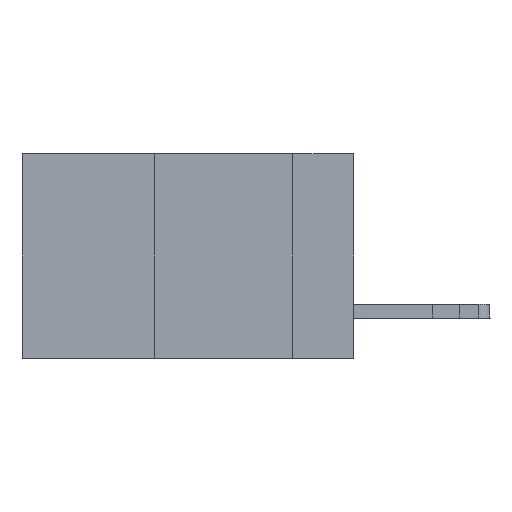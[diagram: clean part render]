
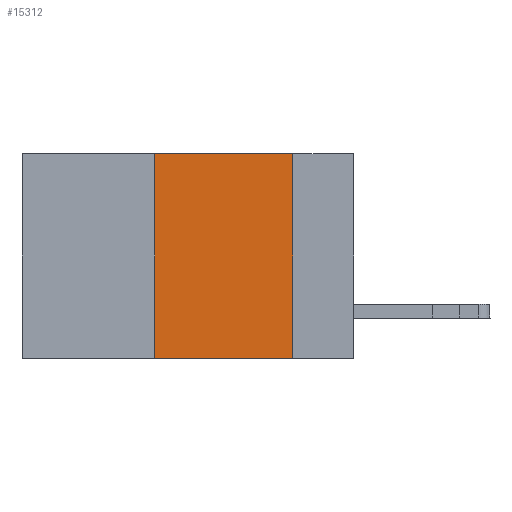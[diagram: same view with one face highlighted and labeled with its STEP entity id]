
A CAD part, left-side view. The second image highlights one B-rep face of the part: STEP entity #15312.
In plain terms, the highlighted planar face has unit normal (-1, 0, 0).
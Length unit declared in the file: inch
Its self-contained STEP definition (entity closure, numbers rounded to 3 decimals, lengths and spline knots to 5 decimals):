
#2094 = DIRECTION ( 'NONE',  ( 1., 0., 0. ) ) ;
#3009 = CARTESIAN_POINT ( 'NONE',  ( 0., 0.11, 0. ) ) ;
#3119 = VECTOR ( 'NONE', #15580, 39.37008 ) ;
#3267 = LINE ( 'NONE', #10671, #11574 ) ;
#3893 = ORIENTED_EDGE ( 'NONE', *, *, #8910, .F. ) ;
#4150 = CARTESIAN_POINT ( 'NONE',  ( 0., 0.6, -0.37 ) ) ;
#4875 = VECTOR ( 'NONE', #9356, 39.37008 ) ;
#5957 = VERTEX_POINT ( 'NONE', #6517 ) ;
#6417 = EDGE_CURVE ( 'NONE', #9310, #8151, #13589, .T. ) ;
#6464 = CARTESIAN_POINT ( 'NONE',  ( 0., 0.36, -0.37 ) ) ;
#6517 = CARTESIAN_POINT ( 'NONE',  ( 0., 0.36, 0. ) ) ;
#7467 = CARTESIAN_POINT ( 'NONE',  ( 0., 0.11, 0. ) ) ;
#8151 = VERTEX_POINT ( 'NONE', #9214 ) ;
#8866 = ORIENTED_EDGE ( 'NONE', *, *, #16537, .F. ) ;
#8910 = EDGE_CURVE ( 'NONE', #5957, #9310, #12838, .T. ) ;
#9214 = CARTESIAN_POINT ( 'NONE',  ( 0., 0.11, -0.37 ) ) ;
#9310 = VERTEX_POINT ( 'NONE', #7467 ) ;
#9356 = DIRECTION ( 'NONE',  ( 0., 0., -1. ) ) ;
#9537 = CARTESIAN_POINT ( 'NONE',  ( 0., 0.6, 0. ) ) ;
#9902 = ORIENTED_EDGE ( 'NONE', *, *, #14294, .T. ) ;
#10671 = CARTESIAN_POINT ( 'NONE',  ( 0., 0.36, 0. ) ) ;
#11574 = VECTOR ( 'NONE', #12287, 39.37008 ) ;
#12052 = CARTESIAN_POINT ( 'NONE',  ( 0., 0.6, 0. ) ) ;
#12287 = DIRECTION ( 'NONE',  ( 0., 0., 1. ) ) ;
#12838 = LINE ( 'NONE', #9537, #16549 ) ;
#13589 = LINE ( 'NONE', #3009, #4875 ) ;
#13662 = DIRECTION ( 'NONE',  ( 0., 0., -1. ) ) ;
#14294 = EDGE_CURVE ( 'NONE', #14515, #8151, #15181, .T. ) ;
#14385 = DIRECTION ( 'NONE',  ( 0., -1., 0. ) ) ;
#14515 = VERTEX_POINT ( 'NONE', #6464 ) ;
#15181 = LINE ( 'NONE', #4150, #3119 ) ;
#15312 = ADVANCED_FACE ( 'NONE', ( #20128 ), #19990, .F. ) ;
#15359 = EDGE_LOOP ( 'NONE', ( #16398, #3893, #8866, #9902 ) ) ;
#15580 = DIRECTION ( 'NONE',  ( 0., -1., 0. ) ) ;
#16398 = ORIENTED_EDGE ( 'NONE', *, *, #6417, .F. ) ;
#16537 = EDGE_CURVE ( 'NONE', #14515, #5957, #3267, .T. ) ;
#16549 = VECTOR ( 'NONE', #14385, 39.37008 ) ;
#19990 = PLANE ( 'NONE',  #20501 ) ;
#20128 = FACE_OUTER_BOUND ( 'NONE', #15359, .T. ) ;
#20501 = AXIS2_PLACEMENT_3D ( 'NONE', #12052, #2094, #13662 ) ;
